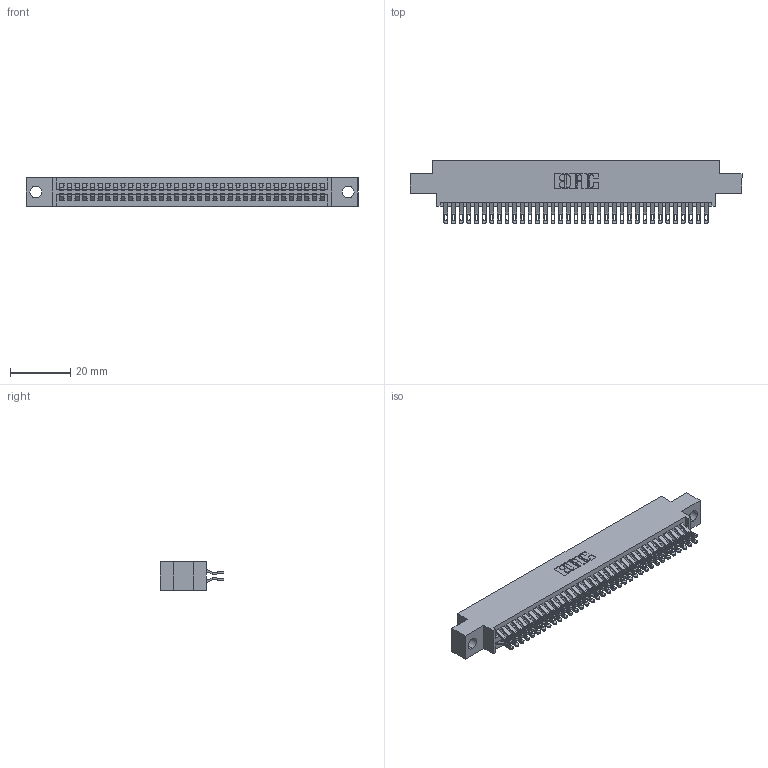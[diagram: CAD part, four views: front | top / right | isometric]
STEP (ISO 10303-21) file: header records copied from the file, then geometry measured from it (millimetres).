
FILE_DESCRIPTION (( 'STEP AP203' ), '1' );
FILE_NAME ('345-070-555-804.STEP', '2018-10-01T09:30:22', ( '' ), ( '' ), 'SwSTEP 2.0', 'SolidWorks 2016', '' );
FILE_SCHEMA (( 'CONFIG_CONTROL_DESIGN' ));
Length unit declared in the file: inch
Products named in the file (3): 345 Part_0.170 Offset - 0.156 Dia-TH; 345-292-001_555 Tail; 345-070-555-804
Assembly tree (71 placements, depth 2):
  345-070-555-804
    345 Part_0.170 Offset - 0.156 Dia-TH
    345-292-001_555 Tail  x70
Bounding box: 110.11 x 21.13 x 9.4 mm (x, y, z)
Volume: 10632.9 mm3; surface area: 16246.5 mm2
Topology: 71 solids, 71 shells, 4050 faces, 12743 edges, 8494 vertices
Faces by surface type: plane 2254, cylinder 1796
Entity records: 28865 total; most frequent: CARTESIAN_POINT 4882, ORIENTED_EDGE 4786, DIRECTION 4281, EDGE_CURVE 2393, VECTOR 2101, LINE 2101, VERTEX_POINT 1594, AXIS2_PLACEMENT_3D 1090
